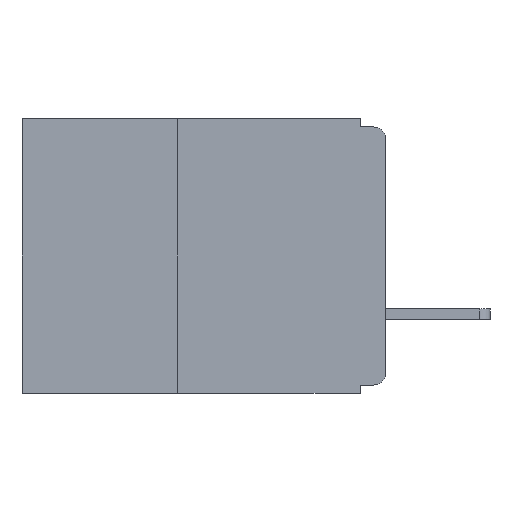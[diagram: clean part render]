
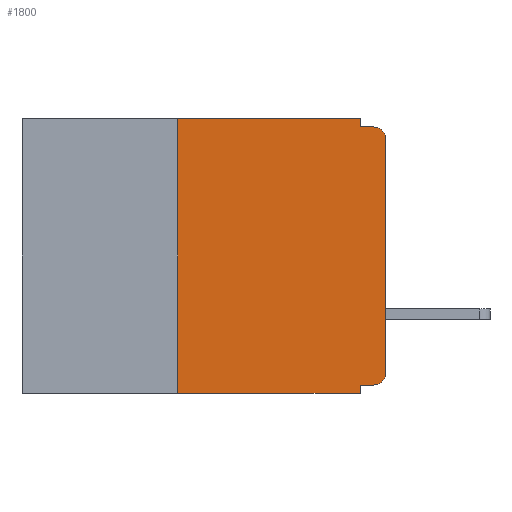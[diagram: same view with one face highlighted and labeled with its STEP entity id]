
A CAD part, left-side view. The second image highlights one B-rep face of the part: STEP entity #1800.
In plain terms, the highlighted planar face has unit normal (-1, 0, 0).
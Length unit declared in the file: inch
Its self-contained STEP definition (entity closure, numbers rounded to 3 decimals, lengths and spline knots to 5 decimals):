
#457 = VERTEX_POINT ( 'NONE', #7103 ) ;
#768 = VERTEX_POINT ( 'NONE', #11471 ) ;
#825 = LINE ( 'NONE', #7188, #4412 ) ;
#935 = AXIS2_PLACEMENT_3D ( 'NONE', #9619, #1543, #10934 ) ;
#1317 = AXIS2_PLACEMENT_3D ( 'NONE', #11465, #6362, #7022 ) ;
#1543 = DIRECTION ( 'NONE',  ( -1., 0., 0. ) ) ;
#1800 = ADVANCED_FACE ( 'NONE', ( #12314 ), #8676, .F. ) ;
#1912 = LINE ( 'NONE', #15365, #12144 ) ;
#2033 = VECTOR ( 'NONE', #15645, 39.37008 ) ;
#2040 = CARTESIAN_POINT ( 'NONE',  ( 0., 0.015, -0.32 ) ) ;
#2200 = VECTOR ( 'NONE', #9431, 39.37008 ) ;
#2305 = CARTESIAN_POINT ( 'NONE',  ( 0., 0.031, -0.01 ) ) ;
#2390 = LINE ( 'NONE', #10271, #9106 ) ;
#2443 = DIRECTION ( 'NONE',  ( 0., 0., -1. ) ) ;
#2447 = DIRECTION ( 'NONE',  ( -1., 0., 0. ) ) ;
#2468 = CARTESIAN_POINT ( 'NONE',  ( 0., 0.015, -0.025 ) ) ;
#3570 = LINE ( 'NONE', #6718, #7122 ) ;
#3730 = CARTESIAN_POINT ( 'NONE',  ( 0., 0.25, -0.33 ) ) ;
#3857 = DIRECTION ( 'NONE',  ( 0., 1., 0. ) ) ;
#4226 = VECTOR ( 'NONE', #7088, 39.37008 ) ;
#4395 = CIRCLE ( 'NONE', #8121, 0.015 ) ;
#4412 = VECTOR ( 'NONE', #7201, 39.37008 ) ;
#5354 = LINE ( 'NONE', #12043, #2200 ) ;
#5616 = ORIENTED_EDGE ( 'NONE', *, *, #13803, .F. ) ;
#5832 = ORIENTED_EDGE ( 'NONE', *, *, #7132, .T. ) ;
#5958 = EDGE_LOOP ( 'NONE', ( #6588, #10749, #15027, #6233, #7237, #14851, #5832, #7102, #5616, #9277 ) ) ;
#6179 = DIRECTION ( 'NONE',  ( 0., -1., 0. ) ) ;
#6233 = ORIENTED_EDGE ( 'NONE', *, *, #12475, .F. ) ;
#6362 = DIRECTION ( 'NONE',  ( 1., 0., 0. ) ) ;
#6468 = LINE ( 'NONE', #9173, #2033 ) ;
#6588 = ORIENTED_EDGE ( 'NONE', *, *, #7178, .T. ) ;
#6718 = CARTESIAN_POINT ( 'NONE',  ( 0., 0., 0. ) ) ;
#6822 = DIRECTION ( 'NONE',  ( 0., 0., 1. ) ) ;
#7018 = VECTOR ( 'NONE', #3857, 39.37008 ) ;
#7022 = DIRECTION ( 'NONE',  ( 0., 0., -1. ) ) ;
#7088 = DIRECTION ( 'NONE',  ( 0., 0., 1. ) ) ;
#7102 = ORIENTED_EDGE ( 'NONE', *, *, #14519, .F. ) ;
#7103 = CARTESIAN_POINT ( 'NONE',  ( 0., 0.031, 0. ) ) ;
#7122 = VECTOR ( 'NONE', #6822, 39.37008 ) ;
#7132 = EDGE_CURVE ( 'NONE', #8022, #16758, #825, .T. ) ;
#7178 = EDGE_CURVE ( 'NONE', #15042, #14379, #3570, .T. ) ;
#7188 = CARTESIAN_POINT ( 'NONE',  ( 0., 0.437, -0.33 ) ) ;
#7201 = DIRECTION ( 'NONE',  ( 0., -1., 0. ) ) ;
#7237 = ORIENTED_EDGE ( 'NONE', *, *, #13899, .F. ) ;
#7425 = LINE ( 'NONE', #11828, #7018 ) ;
#7606 = EDGE_CURVE ( 'NONE', #14379, #10411, #4395, .T. ) ;
#7631 = VERTEX_POINT ( 'NONE', #2305 ) ;
#7757 = LINE ( 'NONE', #9809, #4226 ) ;
#8022 = VERTEX_POINT ( 'NONE', #3730 ) ;
#8121 = AXIS2_PLACEMENT_3D ( 'NONE', #2468, #2447, #2443 ) ;
#8491 = VERTEX_POINT ( 'NONE', #16062 ) ;
#8676 = PLANE ( 'NONE',  #1317 ) ;
#9106 = VECTOR ( 'NONE', #11573, 39.37008 ) ;
#9173 = CARTESIAN_POINT ( 'NONE',  ( 0., 0.031, 0. ) ) ;
#9277 = ORIENTED_EDGE ( 'NONE', *, *, #16700, .T. ) ;
#9431 = DIRECTION ( 'NONE',  ( 0., -1., 0. ) ) ;
#9619 = CARTESIAN_POINT ( 'NONE',  ( 0., 0.015, -0.305 ) ) ;
#9809 = CARTESIAN_POINT ( 'NONE',  ( 0., 0.25, -0.33 ) ) ;
#9859 = EDGE_CURVE ( 'NONE', #8022, #8491, #7757, .T. ) ;
#10271 = CARTESIAN_POINT ( 'NONE',  ( 0., 0.031, -0.33 ) ) ;
#10411 = VERTEX_POINT ( 'NONE', #10881 ) ;
#10749 = ORIENTED_EDGE ( 'NONE', *, *, #7606, .T. ) ;
#10881 = CARTESIAN_POINT ( 'NONE',  ( 0., 0.015, -0.01 ) ) ;
#10934 = DIRECTION ( 'NONE',  ( 0., 0., -1. ) ) ;
#11465 = CARTESIAN_POINT ( 'NONE',  ( 0., 0.437, 0. ) ) ;
#11471 = CARTESIAN_POINT ( 'NONE',  ( 0., 0.031, -0.32 ) ) ;
#11573 = DIRECTION ( 'NONE',  ( 0., 0., -1. ) ) ;
#11828 = CARTESIAN_POINT ( 'NONE',  ( 0., 0., -0.32 ) ) ;
#12043 = CARTESIAN_POINT ( 'NONE',  ( 0., 0.437, 0. ) ) ;
#12144 = VECTOR ( 'NONE', #6179, 39.37008 ) ;
#12314 = FACE_OUTER_BOUND ( 'NONE', #5958, .T. ) ;
#12475 = EDGE_CURVE ( 'NONE', #457, #7631, #6468, .T. ) ;
#13187 = CARTESIAN_POINT ( 'NONE',  ( 0., 0., -0.025 ) ) ;
#13597 = CARTESIAN_POINT ( 'NONE',  ( 0., 0.031, -0.33 ) ) ;
#13803 = EDGE_CURVE ( 'NONE', #16315, #768, #7425, .T. ) ;
#13878 = CARTESIAN_POINT ( 'NONE',  ( 0., 0., -0.305 ) ) ;
#13899 = EDGE_CURVE ( 'NONE', #8491, #457, #5354, .T. ) ;
#14337 = CIRCLE ( 'NONE', #935, 0.015 ) ;
#14379 = VERTEX_POINT ( 'NONE', #13187 ) ;
#14519 = EDGE_CURVE ( 'NONE', #768, #16758, #2390, .T. ) ;
#14851 = ORIENTED_EDGE ( 'NONE', *, *, #9859, .F. ) ;
#15027 = ORIENTED_EDGE ( 'NONE', *, *, #15751, .F. ) ;
#15042 = VERTEX_POINT ( 'NONE', #13878 ) ;
#15365 = CARTESIAN_POINT ( 'NONE',  ( 0., 0., -0.01 ) ) ;
#15645 = DIRECTION ( 'NONE',  ( 0., 0., -1. ) ) ;
#15751 = EDGE_CURVE ( 'NONE', #7631, #10411, #1912, .T. ) ;
#16062 = CARTESIAN_POINT ( 'NONE',  ( 0., 0.25, 0. ) ) ;
#16315 = VERTEX_POINT ( 'NONE', #2040 ) ;
#16700 = EDGE_CURVE ( 'NONE', #16315, #15042, #14337, .T. ) ;
#16758 = VERTEX_POINT ( 'NONE', #13597 ) ;
